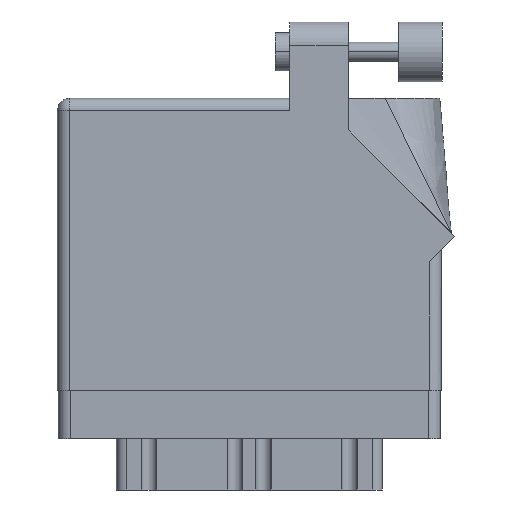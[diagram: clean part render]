
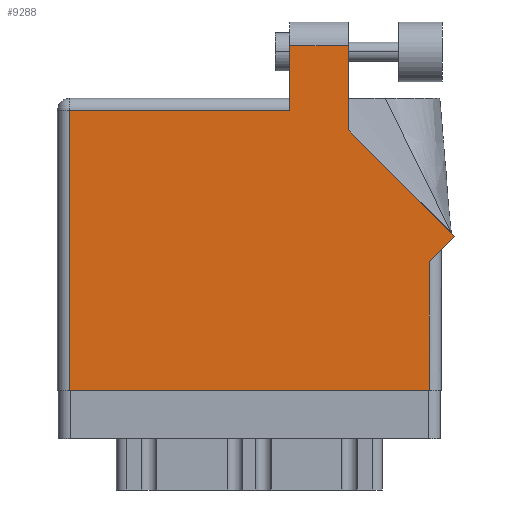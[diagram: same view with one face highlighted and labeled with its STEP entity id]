
A CAD part, front view. The second image highlights one B-rep face of the part: STEP entity #9288.
In plain terms, the highlighted face is planar.
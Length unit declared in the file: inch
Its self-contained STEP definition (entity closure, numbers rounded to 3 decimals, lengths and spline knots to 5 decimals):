
#586 = CARTESIAN_POINT ( 'NONE',  ( 0.062, 0., 0. ) ) ;
#787 = DIRECTION ( 'NONE',  ( 0., 1., 0. ) ) ;
#2057 = FACE_OUTER_BOUND ( 'NONE', #9119, .T. ) ;
#2176 = ORIENTED_EDGE ( 'NONE', *, *, #14954, .T. ) ;
#2713 = DIRECTION ( 'NONE',  ( 0., -1., 0. ) ) ;
#3430 = CARTESIAN_POINT ( 'NONE',  ( 1.524, 1.36442, 0. ) ) ;
#3475 = VECTOR ( 'NONE', #29302, 39.37008 ) ;
#3942 = DIRECTION ( 'NONE',  ( -1., 0., 0. ) ) ;
#4498 = VERTEX_POINT ( 'NONE', #29350 ) ;
#4536 = VERTEX_POINT ( 'NONE', #7365 ) ;
#4648 = DIRECTION ( 'NONE',  ( 1., 0., 0. ) ) ;
#5472 = VECTOR ( 'NONE', #24188, 39.37008 ) ;
#6651 = ORIENTED_EDGE ( 'NONE', *, *, #27225, .T. ) ;
#7365 = CARTESIAN_POINT ( 'NONE',  ( 1.217, 1.805, 0. ) ) ;
#7737 = CARTESIAN_POINT ( 'NONE',  ( 2.08071, 0.80771, 0. ) ) ;
#7951 = VECTOR ( 'NONE', #11858, 39.37008 ) ;
#7992 = VERTEX_POINT ( 'NONE', #26399 ) ;
#8036 = VECTOR ( 'NONE', #29768, 39.37008 ) ;
#8137 = CARTESIAN_POINT ( 'NONE',  ( 1.948, 0.675, 0. ) ) ;
#8401 = EDGE_CURVE ( 'NONE', #8540, #15031, #16118, .T. ) ;
#8540 = VERTEX_POINT ( 'NONE', #22407 ) ;
#9119 = EDGE_LOOP ( 'NONE', ( #2176, #6651, #18791, #32856, #9298, #29787, #12131, #34237, #21409 ) ) ;
#9288 = ADVANCED_FACE ( 'NONE', ( #2057 ), #15631, .F. ) ;
#9298 = ORIENTED_EDGE ( 'NONE', *, *, #8401, .T. ) ;
#9659 = CARTESIAN_POINT ( 'NONE',  ( 2.08071, 0.80771, 0. ) ) ;
#9986 = VERTEX_POINT ( 'NONE', #17298 ) ;
#11115 = CARTESIAN_POINT ( 'NONE',  ( 2.01, 0.737, 0. ) ) ;
#11858 = DIRECTION ( 'NONE',  ( 0., -1., 0. ) ) ;
#12131 = ORIENTED_EDGE ( 'NONE', *, *, #20951, .T. ) ;
#12582 = CARTESIAN_POINT ( 'NONE',  ( 0., 0., 0. ) ) ;
#12808 = CARTESIAN_POINT ( 'NONE',  ( 0., 1.53, 0. ) ) ;
#13729 = EDGE_CURVE ( 'NONE', #15031, #7992, #15399, .T. ) ;
#13794 = EDGE_CURVE ( 'NONE', #18963, #8540, #17320, .T. ) ;
#14473 = CARTESIAN_POINT ( 'NONE',  ( 1.217, 1.53, 0. ) ) ;
#14954 = EDGE_CURVE ( 'NONE', #9986, #4498, #27543, .T. ) ;
#15031 = VERTEX_POINT ( 'NONE', #17858 ) ;
#15399 = LINE ( 'NONE', #12582, #28140 ) ;
#15631 = PLANE ( 'NONE',  #19356 ) ;
#16103 = LINE ( 'NONE', #16446, #3475 ) ;
#16118 = LINE ( 'NONE', #586, #26687 ) ;
#16446 = CARTESIAN_POINT ( 'NONE',  ( 1.217, 1.805, 0. ) ) ;
#16694 = EDGE_CURVE ( 'NONE', #4536, #18963, #16957, .T. ) ;
#16957 = LINE ( 'NONE', #14473, #7951 ) ;
#17298 = CARTESIAN_POINT ( 'NONE',  ( 1.524, 1.36442, 0. ) ) ;
#17320 = LINE ( 'NONE', #20489, #24213 ) ;
#17561 = LINE ( 'NONE', #9659, #29420 ) ;
#17711 = VERTEX_POINT ( 'NONE', #7737 ) ;
#17858 = CARTESIAN_POINT ( 'NONE',  ( 0.062, 0., 0. ) ) ;
#18441 = DIRECTION ( 'NONE',  ( 0., 0., -1. ) ) ;
#18791 = ORIENTED_EDGE ( 'NONE', *, *, #16694, .T. ) ;
#18907 = LINE ( 'NONE', #21544, #5472 ) ;
#18963 = VERTEX_POINT ( 'NONE', #20015 ) ;
#19031 = LINE ( 'NONE', #11115, #8036 ) ;
#19356 = AXIS2_PLACEMENT_3D ( 'NONE', #12808, #18441, #26347 ) ;
#20015 = CARTESIAN_POINT ( 'NONE',  ( 1.217, 1.468, 0. ) ) ;
#20489 = CARTESIAN_POINT ( 'NONE',  ( 0., 1.468, 0. ) ) ;
#20951 = EDGE_CURVE ( 'NONE', #7992, #33699, #18907, .T. ) ;
#21409 = ORIENTED_EDGE ( 'NONE', *, *, #26638, .T. ) ;
#21544 = CARTESIAN_POINT ( 'NONE',  ( 1.948, 0.737, 0. ) ) ;
#22407 = CARTESIAN_POINT ( 'NONE',  ( 0.062, 1.468, 0. ) ) ;
#24188 = DIRECTION ( 'NONE',  ( 0., 1., 0. ) ) ;
#24213 = VECTOR ( 'NONE', #3942, 39.37008 ) ;
#26347 = DIRECTION ( 'NONE',  ( -1., 0., 0. ) ) ;
#26399 = CARTESIAN_POINT ( 'NONE',  ( 1.948, 0., 0. ) ) ;
#26638 = EDGE_CURVE ( 'NONE', #17711, #9986, #17561, .T. ) ;
#26687 = VECTOR ( 'NONE', #2713, 39.37008 ) ;
#27225 = EDGE_CURVE ( 'NONE', #4498, #4536, #16103, .T. ) ;
#27543 = LINE ( 'NONE', #3430, #28062 ) ;
#27693 = EDGE_CURVE ( 'NONE', #33699, #17711, #19031, .T. ) ;
#28062 = VECTOR ( 'NONE', #787, 39.37008 ) ;
#28140 = VECTOR ( 'NONE', #4648, 39.37008 ) ;
#29302 = DIRECTION ( 'NONE',  ( -1., 0., 0. ) ) ;
#29350 = CARTESIAN_POINT ( 'NONE',  ( 1.524, 1.805, 0. ) ) ;
#29420 = VECTOR ( 'NONE', #33234, 39.37008 ) ;
#29768 = DIRECTION ( 'NONE',  ( 0.707, 0.707, 0. ) ) ;
#29787 = ORIENTED_EDGE ( 'NONE', *, *, #13729, .T. ) ;
#32856 = ORIENTED_EDGE ( 'NONE', *, *, #13794, .T. ) ;
#33234 = DIRECTION ( 'NONE',  ( -0.707, 0.707, 0. ) ) ;
#33699 = VERTEX_POINT ( 'NONE', #8137 ) ;
#34237 = ORIENTED_EDGE ( 'NONE', *, *, #27693, .T. ) ;
